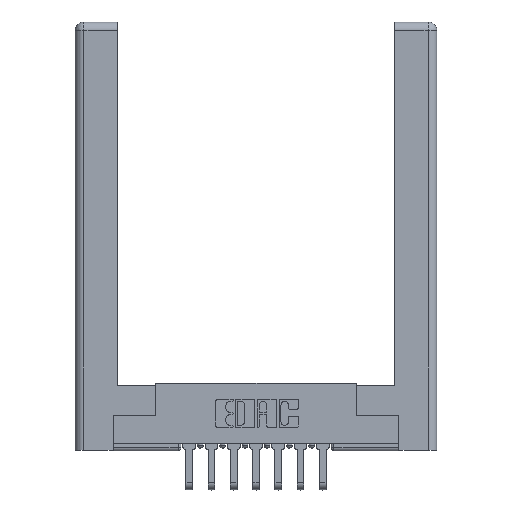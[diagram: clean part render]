
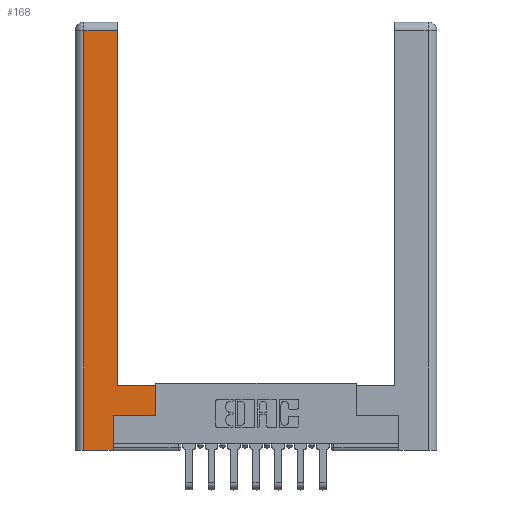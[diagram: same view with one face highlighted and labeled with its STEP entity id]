
A CAD part, top view. The second image highlights one B-rep face of the part: STEP entity #168.
In plain terms, the highlighted planar face has unit normal (0, 0, 1).
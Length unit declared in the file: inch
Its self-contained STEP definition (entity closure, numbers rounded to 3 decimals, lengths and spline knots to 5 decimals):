
#147 = EDGE_CURVE ( 'NONE', #11679, #634, #12254, .T. ) ;
#168 = ADVANCED_FACE ( 'NONE', ( #14212 ), #1552, .F. ) ;
#231 = CARTESIAN_POINT ( 'NONE',  ( 0.0615, 0., 0. ) ) ;
#271 = VECTOR ( 'NONE', #10509, 39.37008 ) ;
#475 = DIRECTION ( 'NONE',  ( 0., 0., -1. ) ) ;
#551 = DIRECTION ( 'NONE',  ( 0., 1., 0. ) ) ;
#634 = VERTEX_POINT ( 'NONE', #1135 ) ;
#1135 = CARTESIAN_POINT ( 'NONE',  ( 0.295, 2.94, 0. ) ) ;
#1169 = CARTESIAN_POINT ( 'NONE',  ( 0.0615, 2.94, 0. ) ) ;
#1308 = CARTESIAN_POINT ( 'NONE',  ( 0.565, 0.45, 0. ) ) ;
#1354 = ORIENTED_EDGE ( 'NONE', *, *, #14429, .T. ) ;
#1388 = LINE ( 'NONE', #12553, #3865 ) ;
#1552 = PLANE ( 'NONE',  #3942 ) ;
#1565 = CARTESIAN_POINT ( 'NONE',  ( 0.295, 0.45, 0. ) ) ;
#1818 = EDGE_CURVE ( 'NONE', #6357, #6901, #1388, .T. ) ;
#1880 = VECTOR ( 'NONE', #4139, 39.37008 ) ;
#2075 = DIRECTION ( 'NONE',  ( 0., 1., 0. ) ) ;
#2094 = ORIENTED_EDGE ( 'NONE', *, *, #1818, .T. ) ;
#2109 = CARTESIAN_POINT ( 'NONE',  ( 0.265, 0., 0. ) ) ;
#2269 = DIRECTION ( 'NONE',  ( 0., -1., 0. ) ) ;
#2491 = VERTEX_POINT ( 'NONE', #1308 ) ;
#2865 = EDGE_CURVE ( 'NONE', #2491, #11679, #11806, .T. ) ;
#3332 = EDGE_CURVE ( 'NONE', #6901, #10139, #14637, .T. ) ;
#3568 = LINE ( 'NONE', #9399, #4630 ) ;
#3865 = VECTOR ( 'NONE', #2269, 39.37008 ) ;
#3942 = AXIS2_PLACEMENT_3D ( 'NONE', #11784, #475, #8428 ) ;
#4139 = DIRECTION ( 'NONE',  ( 1., 0., 0. ) ) ;
#4229 = EDGE_CURVE ( 'NONE', #12890, #5759, #14433, .T. ) ;
#4469 = VECTOR ( 'NONE', #2075, 39.37008 ) ;
#4630 = VECTOR ( 'NONE', #12960, 39.37008 ) ;
#4889 = CARTESIAN_POINT ( 'NONE',  ( 0.565, 0.45, 0. ) ) ;
#5759 = VERTEX_POINT ( 'NONE', #13611 ) ;
#5975 = EDGE_LOOP ( 'NONE', ( #10143, #8437, #2094, #6207, #13666, #7590, #1354, #11549 ) ) ;
#6207 = ORIENTED_EDGE ( 'NONE', *, *, #3332, .T. ) ;
#6329 = CARTESIAN_POINT ( 'NONE',  ( 0.565, 0.245, 0. ) ) ;
#6357 = VERTEX_POINT ( 'NONE', #1169 ) ;
#6627 = LINE ( 'NONE', #9282, #271 ) ;
#6901 = VERTEX_POINT ( 'NONE', #231 ) ;
#7161 = LINE ( 'NONE', #4889, #12810 ) ;
#7590 = ORIENTED_EDGE ( 'NONE', *, *, #4229, .T. ) ;
#8428 = DIRECTION ( 'NONE',  ( -1., 0., 0. ) ) ;
#8437 = ORIENTED_EDGE ( 'NONE', *, *, #14331, .T. ) ;
#8798 = VECTOR ( 'NONE', #12227, 39.37008 ) ;
#9282 = CARTESIAN_POINT ( 'NONE',  ( 0.0615, 2.94, 0. ) ) ;
#9399 = CARTESIAN_POINT ( 'NONE',  ( 0.265, 0.245, 0. ) ) ;
#9583 = DIRECTION ( 'NONE',  ( 1., 0., 0. ) ) ;
#9663 = CARTESIAN_POINT ( 'NONE',  ( 0.265, 0., 0. ) ) ;
#9915 = CARTESIAN_POINT ( 'NONE',  ( 0.295, 3., 0. ) ) ;
#10139 = VERTEX_POINT ( 'NONE', #2109 ) ;
#10143 = ORIENTED_EDGE ( 'NONE', *, *, #147, .T. ) ;
#10509 = DIRECTION ( 'NONE',  ( -1., 0., 0. ) ) ;
#10996 = CARTESIAN_POINT ( 'NONE',  ( 0.265, 0.245, 0. ) ) ;
#11549 = ORIENTED_EDGE ( 'NONE', *, *, #2865, .T. ) ;
#11679 = VERTEX_POINT ( 'NONE', #1565 ) ;
#11784 = CARTESIAN_POINT ( 'NONE',  ( 0., 0., 0. ) ) ;
#11806 = LINE ( 'NONE', #13164, #8798 ) ;
#12067 = EDGE_CURVE ( 'NONE', #10139, #12890, #3568, .T. ) ;
#12227 = DIRECTION ( 'NONE',  ( -1., 0., 0. ) ) ;
#12254 = LINE ( 'NONE', #9915, #4469 ) ;
#12553 = CARTESIAN_POINT ( 'NONE',  ( 0.0615, 0., 0. ) ) ;
#12810 = VECTOR ( 'NONE', #551, 39.37008 ) ;
#12841 = VECTOR ( 'NONE', #9583, 39.37008 ) ;
#12890 = VERTEX_POINT ( 'NONE', #10996 ) ;
#12960 = DIRECTION ( 'NONE',  ( 0., 1., 0. ) ) ;
#13164 = CARTESIAN_POINT ( 'NONE',  ( 0.295, 0.45, 0. ) ) ;
#13611 = CARTESIAN_POINT ( 'NONE',  ( 0.565, 0.245, 0. ) ) ;
#13666 = ORIENTED_EDGE ( 'NONE', *, *, #12067, .T. ) ;
#14212 = FACE_OUTER_BOUND ( 'NONE', #5975, .T. ) ;
#14331 = EDGE_CURVE ( 'NONE', #634, #6357, #6627, .T. ) ;
#14429 = EDGE_CURVE ( 'NONE', #5759, #2491, #7161, .T. ) ;
#14433 = LINE ( 'NONE', #6329, #12841 ) ;
#14637 = LINE ( 'NONE', #9663, #1880 ) ;
